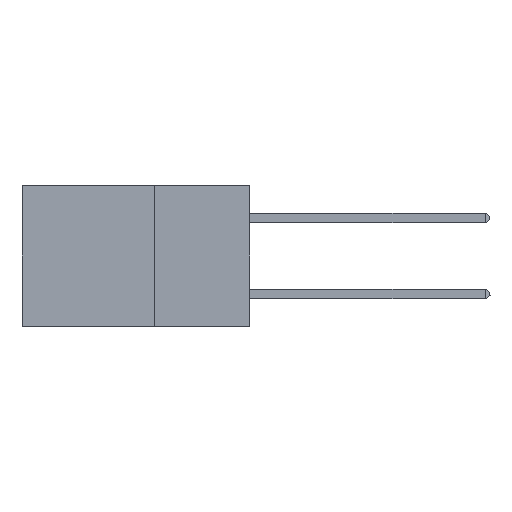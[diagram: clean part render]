
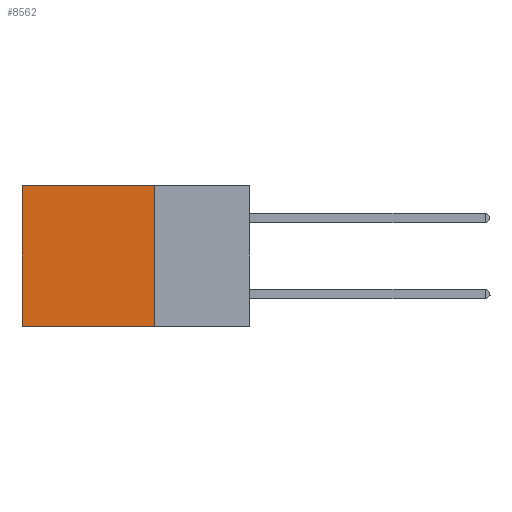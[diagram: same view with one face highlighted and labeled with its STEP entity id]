
A CAD part, left-side view. The second image highlights one B-rep face of the part: STEP entity #8562.
In plain terms, the highlighted planar face has unit normal (-1, 0, 0).
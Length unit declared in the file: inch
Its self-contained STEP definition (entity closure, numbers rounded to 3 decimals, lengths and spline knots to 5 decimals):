
#3667 = ORIENTED_EDGE ( 'NONE', *, *, #12780, .F. ) ;
#4467 = DIRECTION ( 'NONE',  ( 0., 0., -1. ) ) ;
#4906 = CARTESIAN_POINT ( 'NONE',  ( 0.2875, 0.25, 0. ) ) ;
#5368 = VECTOR ( 'NONE', #7826, 39.37008 ) ;
#6663 = DIRECTION ( 'NONE',  ( 0., 0., -1. ) ) ;
#7082 = VERTEX_POINT ( 'NONE', #33991 ) ;
#7110 = CARTESIAN_POINT ( 'NONE',  ( 0.2875, 0.25, -0.37 ) ) ;
#7705 = LINE ( 'NONE', #21685, #9976 ) ;
#7826 = DIRECTION ( 'NONE',  ( 0., 0., -1. ) ) ;
#8042 = LINE ( 'NONE', #35127, #5368 ) ;
#8562 = ADVANCED_FACE ( 'NONE', ( #34877 ), #8657, .F. ) ;
#8657 = PLANE ( 'NONE',  #37730 ) ;
#9795 = VERTEX_POINT ( 'NONE', #10081 ) ;
#9976 = VECTOR ( 'NONE', #11683, 39.37008 ) ;
#10081 = CARTESIAN_POINT ( 'NONE',  ( 0.2875, 0.25, 0. ) ) ;
#11105 = DIRECTION ( 'NONE',  ( 0., 1., 0. ) ) ;
#11683 = DIRECTION ( 'NONE',  ( 0., 1., 0. ) ) ;
#12780 = EDGE_CURVE ( 'NONE', #7082, #36033, #24437, .T. ) ;
#18880 = DIRECTION ( 'NONE',  ( 1., 0., 0. ) ) ;
#20206 = ORIENTED_EDGE ( 'NONE', *, *, #35350, .T. ) ;
#20744 = ORIENTED_EDGE ( 'NONE', *, *, #38654, .F. ) ;
#21495 = VERTEX_POINT ( 'NONE', #23285 ) ;
#21685 = CARTESIAN_POINT ( 'NONE',  ( 0.2875, 0.25, 0. ) ) ;
#23285 = CARTESIAN_POINT ( 'NONE',  ( 0.2875, 0.6, 0. ) ) ;
#23536 = CARTESIAN_POINT ( 'NONE',  ( 0.2875, 0.25, 0. ) ) ;
#24437 = LINE ( 'NONE', #7110, #29391 ) ;
#24863 = EDGE_LOOP ( 'NONE', ( #20206, #3667, #20744, #38386 ) ) ;
#29391 = VECTOR ( 'NONE', #11105, 39.37008 ) ;
#33991 = CARTESIAN_POINT ( 'NONE',  ( 0.2875, 0.25, -0.37 ) ) ;
#34174 = LINE ( 'NONE', #23536, #43038 ) ;
#34877 = FACE_OUTER_BOUND ( 'NONE', #24863, .T. ) ;
#35127 = CARTESIAN_POINT ( 'NONE',  ( 0.2875, 0.6, 0. ) ) ;
#35350 = EDGE_CURVE ( 'NONE', #21495, #36033, #8042, .T. ) ;
#35649 = CARTESIAN_POINT ( 'NONE',  ( 0.2875, 0.6, -0.37 ) ) ;
#36033 = VERTEX_POINT ( 'NONE', #35649 ) ;
#37730 = AXIS2_PLACEMENT_3D ( 'NONE', #4906, #18880, #4467 ) ;
#38386 = ORIENTED_EDGE ( 'NONE', *, *, #42954, .T. ) ;
#38654 = EDGE_CURVE ( 'NONE', #9795, #7082, #34174, .T. ) ;
#42954 = EDGE_CURVE ( 'NONE', #9795, #21495, #7705, .T. ) ;
#43038 = VECTOR ( 'NONE', #6663, 39.37008 ) ;
